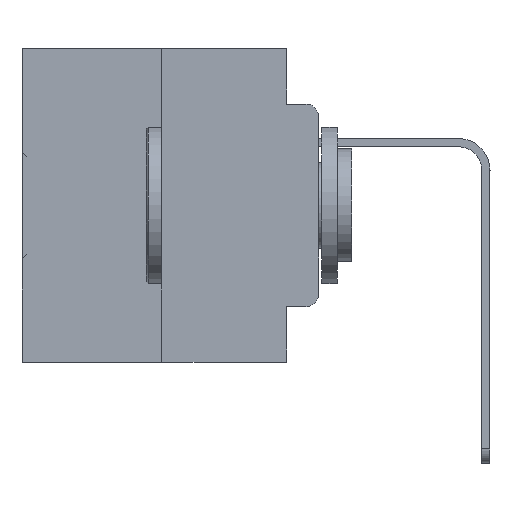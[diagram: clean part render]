
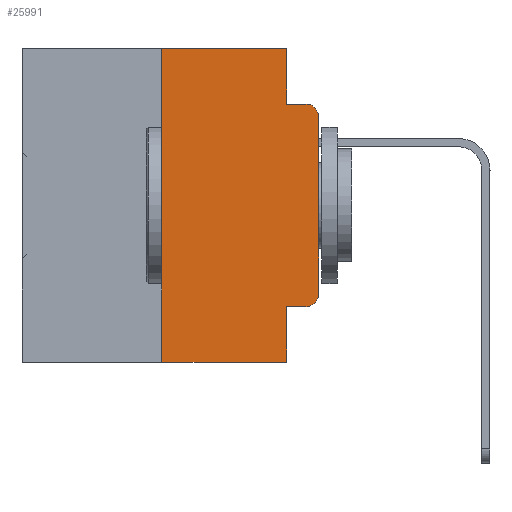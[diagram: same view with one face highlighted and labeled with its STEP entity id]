
A CAD part, left-side view. The second image highlights one B-rep face of the part: STEP entity #25991.
In plain terms, the highlighted planar face has unit normal (-1, 0, 0).
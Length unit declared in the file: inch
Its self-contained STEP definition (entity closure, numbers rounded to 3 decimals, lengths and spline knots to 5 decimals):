
#176 = AXIS2_PLACEMENT_3D ( 'NONE', #2552, #21409, #7975 ) ;
#626 = EDGE_LOOP ( 'NONE', ( #2016, #33651, #13799, #17463, #16839, #22960, #14524, #15036, #4109, #10257 ) ) ;
#665 = CARTESIAN_POINT ( 'NONE',  ( 0., 0.051, -0.0885 ) ) ;
#982 = LINE ( 'NONE', #12091, #18288 ) ;
#1175 = VECTOR ( 'NONE', #27946, 39.37008 ) ;
#1866 = VERTEX_POINT ( 'NONE', #28704 ) ;
#2016 = ORIENTED_EDGE ( 'NONE', *, *, #30936, .T. ) ;
#2552 = CARTESIAN_POINT ( 'NONE',  ( 0., 0.02, -0.3915 ) ) ;
#2764 = EDGE_CURVE ( 'NONE', #13316, #27605, #5503, .T. ) ;
#3281 = LINE ( 'NONE', #665, #1175 ) ;
#4109 = ORIENTED_EDGE ( 'NONE', *, *, #9525, .T. ) ;
#5287 = CARTESIAN_POINT ( 'NONE',  ( 0., 0.02, -0.1085 ) ) ;
#5503 = LINE ( 'NONE', #26175, #31302 ) ;
#6179 = CARTESIAN_POINT ( 'NONE',  ( 0., 0.051, -0.5 ) ) ;
#6330 = CARTESIAN_POINT ( 'NONE',  ( 0., 0.051, 0. ) ) ;
#7119 = CARTESIAN_POINT ( 'NONE',  ( 0., 0.051, -0.4115 ) ) ;
#7975 = DIRECTION ( 'NONE',  ( 0., 0., -1. ) ) ;
#8788 = EDGE_CURVE ( 'NONE', #32631, #30736, #3281, .T. ) ;
#9525 = EDGE_CURVE ( 'NONE', #12043, #1866, #14627, .T. ) ;
#9652 = DIRECTION ( 'NONE',  ( 0., 0., 1. ) ) ;
#9723 = DIRECTION ( 'NONE',  ( 0., -1., 0. ) ) ;
#10257 = ORIENTED_EDGE ( 'NONE', *, *, #28693, .T. ) ;
#11099 = DIRECTION ( 'NONE',  ( 0., -1., 0. ) ) ;
#11129 = DIRECTION ( 'NONE',  ( 0., 0., -1. ) ) ;
#11864 = VECTOR ( 'NONE', #9652, 39.37008 ) ;
#12043 = VERTEX_POINT ( 'NONE', #16208 ) ;
#12091 = CARTESIAN_POINT ( 'NONE',  ( 0., 0.051, 0. ) ) ;
#12408 = DIRECTION ( 'NONE',  ( 0., -1., 0. ) ) ;
#12711 = LINE ( 'NONE', #17571, #11864 ) ;
#12975 = DIRECTION ( 'NONE',  ( 0., 0., -1. ) ) ;
#13316 = VERTEX_POINT ( 'NONE', #30057 ) ;
#13423 = PLANE ( 'NONE',  #32905 ) ;
#13437 = CARTESIAN_POINT ( 'NONE',  ( 0., 0.02, -0.0885 ) ) ;
#13799 = ORIENTED_EDGE ( 'NONE', *, *, #8788, .F. ) ;
#14524 = ORIENTED_EDGE ( 'NONE', *, *, #21039, .T. ) ;
#14627 = LINE ( 'NONE', #7119, #28157 ) ;
#15036 = ORIENTED_EDGE ( 'NONE', *, *, #25142, .F. ) ;
#15494 = CARTESIAN_POINT ( 'NONE',  ( 0., 0.25, 0. ) ) ;
#15934 = CARTESIAN_POINT ( 'NONE',  ( 0., 0.473, 0. ) ) ;
#16208 = CARTESIAN_POINT ( 'NONE',  ( 0., 0.051, -0.4115 ) ) ;
#16479 = VERTEX_POINT ( 'NONE', #32918 ) ;
#16623 = VECTOR ( 'NONE', #33069, 39.37008 ) ;
#16839 = ORIENTED_EDGE ( 'NONE', *, *, #25525, .F. ) ;
#17446 = VECTOR ( 'NONE', #12408, 39.37008 ) ;
#17463 = ORIENTED_EDGE ( 'NONE', *, *, #33155, .F. ) ;
#17571 = CARTESIAN_POINT ( 'NONE',  ( 0., 0., 0. ) ) ;
#18288 = VECTOR ( 'NONE', #11129, 39.37008 ) ;
#21039 = EDGE_CURVE ( 'NONE', #13316, #27393, #24618, .T. ) ;
#21193 = DIRECTION ( 'NONE',  ( 1., 0., 0. ) ) ;
#21326 = EDGE_CURVE ( 'NONE', #16479, #30736, #29230, .T. ) ;
#21409 = DIRECTION ( 'NONE',  ( -1., 0., 0. ) ) ;
#22873 = CARTESIAN_POINT ( 'NONE',  ( 0., 0.473, -0.5 ) ) ;
#22960 = ORIENTED_EDGE ( 'NONE', *, *, #2764, .F. ) ;
#23157 = VERTEX_POINT ( 'NONE', #6330 ) ;
#24153 = DIRECTION ( 'NONE',  ( -1., 0., 0. ) ) ;
#24189 = LINE ( 'NONE', #25296, #16623 ) ;
#24618 = LINE ( 'NONE', #22873, #17446 ) ;
#25142 = EDGE_CURVE ( 'NONE', #12043, #27393, #982, .T. ) ;
#25296 = CARTESIAN_POINT ( 'NONE',  ( 0., 0.051, 0. ) ) ;
#25525 = EDGE_CURVE ( 'NONE', #27605, #23157, #26985, .T. ) ;
#25991 = ADVANCED_FACE ( 'NONE', ( #30762 ), #13423, .F. ) ;
#26175 = CARTESIAN_POINT ( 'NONE',  ( 0., 0.25, 0. ) ) ;
#26985 = LINE ( 'NONE', #29518, #28668 ) ;
#27058 = CARTESIAN_POINT ( 'NONE',  ( 0., 0., -0.3915 ) ) ;
#27393 = VERTEX_POINT ( 'NONE', #6179 ) ;
#27605 = VERTEX_POINT ( 'NONE', #15494 ) ;
#27946 = DIRECTION ( 'NONE',  ( 0., -1., 0. ) ) ;
#28157 = VECTOR ( 'NONE', #9723, 39.37008 ) ;
#28668 = VECTOR ( 'NONE', #11099, 39.37008 ) ;
#28693 = EDGE_CURVE ( 'NONE', #1866, #31922, #30284, .T. ) ;
#28704 = CARTESIAN_POINT ( 'NONE',  ( 0., 0.02, -0.4115 ) ) ;
#29230 = CIRCLE ( 'NONE', #32591, 0.02 ) ;
#29518 = CARTESIAN_POINT ( 'NONE',  ( 0., 0.473, 0. ) ) ;
#30048 = DIRECTION ( 'NONE',  ( 0., 0., -1. ) ) ;
#30057 = CARTESIAN_POINT ( 'NONE',  ( 0., 0.25, -0.5 ) ) ;
#30284 = CIRCLE ( 'NONE', #176, 0.02 ) ;
#30377 = CARTESIAN_POINT ( 'NONE',  ( 0., 0.051, -0.0885 ) ) ;
#30736 = VERTEX_POINT ( 'NONE', #13437 ) ;
#30762 = FACE_OUTER_BOUND ( 'NONE', #626, .T. ) ;
#30936 = EDGE_CURVE ( 'NONE', #31922, #16479, #12711, .T. ) ;
#31302 = VECTOR ( 'NONE', #33951, 39.37008 ) ;
#31922 = VERTEX_POINT ( 'NONE', #27058 ) ;
#32591 = AXIS2_PLACEMENT_3D ( 'NONE', #5287, #24153, #30048 ) ;
#32631 = VERTEX_POINT ( 'NONE', #30377 ) ;
#32905 = AXIS2_PLACEMENT_3D ( 'NONE', #15934, #21193, #12975 ) ;
#32918 = CARTESIAN_POINT ( 'NONE',  ( 0., 0., -0.1085 ) ) ;
#33069 = DIRECTION ( 'NONE',  ( 0., 0., -1. ) ) ;
#33155 = EDGE_CURVE ( 'NONE', #23157, #32631, #24189, .T. ) ;
#33651 = ORIENTED_EDGE ( 'NONE', *, *, #21326, .T. ) ;
#33951 = DIRECTION ( 'NONE',  ( 0., 0., 1. ) ) ;
